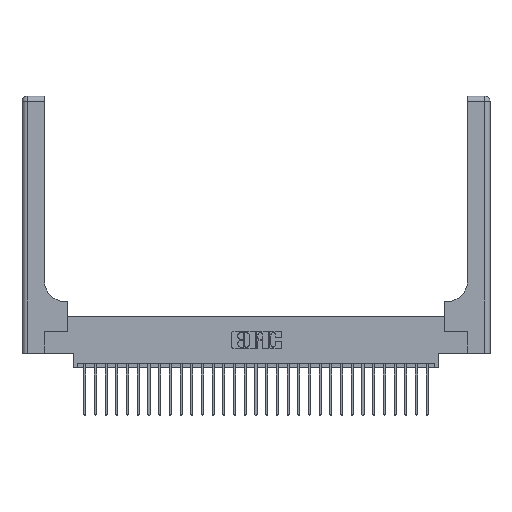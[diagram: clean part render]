
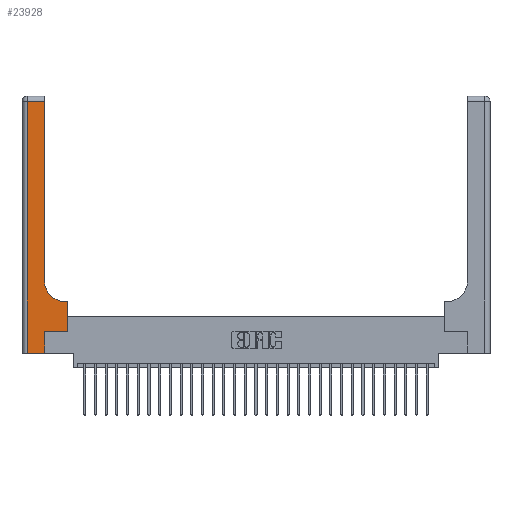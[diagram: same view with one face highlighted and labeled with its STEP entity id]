
A CAD part, top view. The second image highlights one B-rep face of the part: STEP entity #23928.
In plain terms, the highlighted planar face has unit normal (0, 0, 1).
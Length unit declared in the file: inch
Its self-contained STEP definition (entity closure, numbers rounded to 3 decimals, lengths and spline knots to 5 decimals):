
#281 = DIRECTION ( 'NONE',  ( -1., 0., 0. ) ) ;
#283 = ORIENTED_EDGE ( 'NONE', *, *, #15971, .T. ) ;
#577 = EDGE_CURVE ( 'NONE', #2498, #22388, #16534, .T. ) ;
#582 = CARTESIAN_POINT ( 'NONE',  ( 0.26, 2.94, 0.37 ) ) ;
#670 = DIRECTION ( 'NONE',  ( 0., 1., 0. ) ) ;
#1109 = VECTOR ( 'NONE', #9265, 39.37008 ) ;
#1599 = DIRECTION ( 'NONE',  ( 1., 0., 0. ) ) ;
#1852 = VERTEX_POINT ( 'NONE', #17956 ) ;
#1959 = ORIENTED_EDGE ( 'NONE', *, *, #20365, .T. ) ;
#2079 = LINE ( 'NONE', #8373, #13591 ) ;
#2154 = VERTEX_POINT ( 'NONE', #25689 ) ;
#2498 = VERTEX_POINT ( 'NONE', #2988 ) ;
#2988 = CARTESIAN_POINT ( 'NONE',  ( 0.265, 0.25, 0.37 ) ) ;
#3334 = DIRECTION ( 'NONE',  ( 0., 0., -1. ) ) ;
#4199 = EDGE_CURVE ( 'NONE', #2154, #2498, #27445, .T. ) ;
#5435 = CARTESIAN_POINT ( 'NONE',  ( 0.265, 0.25, 0.37 ) ) ;
#5574 = CARTESIAN_POINT ( 'NONE',  ( 0., 0., 0.37 ) ) ;
#6510 = CARTESIAN_POINT ( 'NONE',  ( 0.265, 0., 0.37 ) ) ;
#8354 = EDGE_LOOP ( 'NONE', ( #23687, #1959, #19269, #25057, #19958, #14822, #16197, #22002, #283 ) ) ;
#8373 = CARTESIAN_POINT ( 'NONE',  ( 0.06, 3., 0.37 ) ) ;
#9025 = DIRECTION ( 'NONE',  ( -1., 0., 0. ) ) ;
#9265 = DIRECTION ( 'NONE',  ( 0., 1., 0. ) ) ;
#9777 = DIRECTION ( 'NONE',  ( 1., 0., 0. ) ) ;
#10795 = VECTOR ( 'NONE', #17295, 39.37008 ) ;
#11946 = CARTESIAN_POINT ( 'NONE',  ( 0., 3., 0.37 ) ) ;
#11974 = LINE ( 'NONE', #15702, #1109 ) ;
#13083 = AXIS2_PLACEMENT_3D ( 'NONE', #11946, #3334, #18484 ) ;
#13141 = LINE ( 'NONE', #13246, #25009 ) ;
#13246 = CARTESIAN_POINT ( 'NONE',  ( 0., 2.94, 0.37 ) ) ;
#13591 = VECTOR ( 'NONE', #23560, 39.37008 ) ;
#13890 = VERTEX_POINT ( 'NONE', #24019 ) ;
#14103 = PLANE ( 'NONE',  #13083 ) ;
#14563 = LINE ( 'NONE', #5574, #21062 ) ;
#14565 = DIRECTION ( 'NONE',  ( 0., 0., -1. ) ) ;
#14822 = ORIENTED_EDGE ( 'NONE', *, *, #577, .T. ) ;
#14941 = FACE_OUTER_BOUND ( 'NONE', #8354, .T. ) ;
#15672 = VERTEX_POINT ( 'NONE', #582 ) ;
#15702 = CARTESIAN_POINT ( 'NONE',  ( 0.528, 0.25, 0.37 ) ) ;
#15815 = CARTESIAN_POINT ( 'NONE',  ( 0.26, 0.85, 0.37 ) ) ;
#15971 = EDGE_CURVE ( 'NONE', #13890, #27092, #25930, .T. ) ;
#16171 = CARTESIAN_POINT ( 'NONE',  ( 0.528, 0.25, 0.37 ) ) ;
#16197 = ORIENTED_EDGE ( 'NONE', *, *, #16341, .T. ) ;
#16341 = EDGE_CURVE ( 'NONE', #22388, #27025, #11974, .T. ) ;
#16397 = AXIS2_PLACEMENT_3D ( 'NONE', #27616, #14565, #1599 ) ;
#16534 = LINE ( 'NONE', #5435, #27426 ) ;
#17295 = DIRECTION ( 'NONE',  ( 0., 1., 0. ) ) ;
#17410 = EDGE_CURVE ( 'NONE', #1852, #19725, #2079, .T. ) ;
#17626 = EDGE_CURVE ( 'NONE', #27025, #13890, #21079, .T. ) ;
#17956 = CARTESIAN_POINT ( 'NONE',  ( 0.06, 2.94, 0.37 ) ) ;
#18484 = DIRECTION ( 'NONE',  ( -1., 0., 0. ) ) ;
#19269 = ORIENTED_EDGE ( 'NONE', *, *, #17410, .T. ) ;
#19709 = VECTOR ( 'NONE', #9025, 39.37008 ) ;
#19725 = VERTEX_POINT ( 'NONE', #21936 ) ;
#19958 = ORIENTED_EDGE ( 'NONE', *, *, #4199, .T. ) ;
#20365 = EDGE_CURVE ( 'NONE', #15672, #1852, #13141, .T. ) ;
#20749 = DIRECTION ( 'NONE',  ( 1., 0., 0. ) ) ;
#21062 = VECTOR ( 'NONE', #20749, 39.37008 ) ;
#21079 = LINE ( 'NONE', #21945, #19709 ) ;
#21936 = CARTESIAN_POINT ( 'NONE',  ( 0.06, 0., 0.37 ) ) ;
#21945 = CARTESIAN_POINT ( 'NONE',  ( 0.26, 0.6, 0.37 ) ) ;
#22002 = ORIENTED_EDGE ( 'NONE', *, *, #17626, .T. ) ;
#22388 = VERTEX_POINT ( 'NONE', #16171 ) ;
#22397 = CARTESIAN_POINT ( 'NONE',  ( 0.26, 3., 0.37 ) ) ;
#22602 = LINE ( 'NONE', #22397, #27713 ) ;
#23560 = DIRECTION ( 'NONE',  ( 0., -1., 0. ) ) ;
#23687 = ORIENTED_EDGE ( 'NONE', *, *, #27093, .T. ) ;
#23928 = ADVANCED_FACE ( 'NONE', ( #14941 ), #14103, .F. ) ;
#24019 = CARTESIAN_POINT ( 'NONE',  ( 0.51, 0.6, 0.37 ) ) ;
#24389 = CARTESIAN_POINT ( 'NONE',  ( 0.528, 0.6, 0.37 ) ) ;
#24565 = EDGE_CURVE ( 'NONE', #19725, #2154, #14563, .T. ) ;
#25009 = VECTOR ( 'NONE', #281, 39.37008 ) ;
#25057 = ORIENTED_EDGE ( 'NONE', *, *, #24565, .T. ) ;
#25689 = CARTESIAN_POINT ( 'NONE',  ( 0.265, 0., 0.37 ) ) ;
#25930 = CIRCLE ( 'NONE', #16397, 0.25 ) ;
#27025 = VERTEX_POINT ( 'NONE', #24389 ) ;
#27092 = VERTEX_POINT ( 'NONE', #15815 ) ;
#27093 = EDGE_CURVE ( 'NONE', #27092, #15672, #22602, .T. ) ;
#27426 = VECTOR ( 'NONE', #9777, 39.37008 ) ;
#27445 = LINE ( 'NONE', #6510, #10795 ) ;
#27616 = CARTESIAN_POINT ( 'NONE',  ( 0.51, 0.85, 0.37 ) ) ;
#27713 = VECTOR ( 'NONE', #670, 39.37008 ) ;
